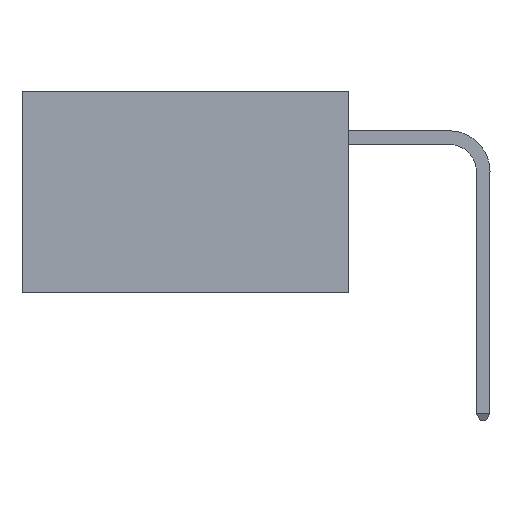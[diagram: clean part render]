
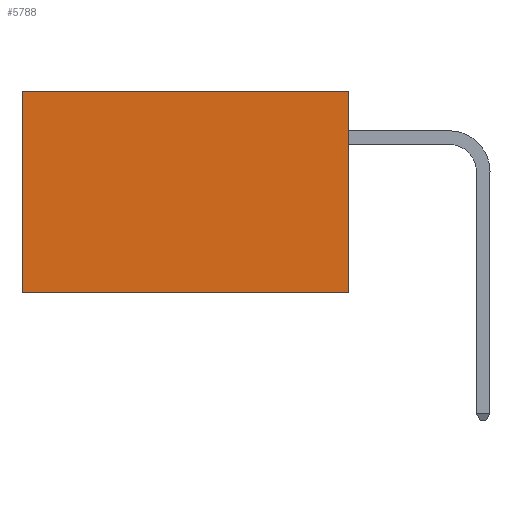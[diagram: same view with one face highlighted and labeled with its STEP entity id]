
A CAD part, left-side view. The second image highlights one B-rep face of the part: STEP entity #5788.
In plain terms, the highlighted planar face has unit normal (-1, 0, 0).
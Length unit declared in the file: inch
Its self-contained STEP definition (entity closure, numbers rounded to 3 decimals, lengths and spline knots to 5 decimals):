
#42 = CARTESIAN_POINT ( 'NONE',  ( 0.2875, 0., 0. ) ) ;
#279 = VERTEX_POINT ( 'NONE', #8494 ) ;
#359 = EDGE_CURVE ( 'NONE', #1684, #279, #5317, .T. ) ;
#578 = VERTEX_POINT ( 'NONE', #4209 ) ;
#621 = CARTESIAN_POINT ( 'NONE',  ( 0.2875, 0., 0. ) ) ;
#719 = DIRECTION ( 'NONE',  ( 0., 1., 0. ) ) ;
#857 = VERTEX_POINT ( 'NONE', #935 ) ;
#935 = CARTESIAN_POINT ( 'NONE',  ( 0.2875, 0.6, -0.37 ) ) ;
#992 = DIRECTION ( 'NONE',  ( 0., 0., -1. ) ) ;
#1509 = VECTOR ( 'NONE', #719, 39.37008 ) ;
#1549 = VECTOR ( 'NONE', #4311, 39.37008 ) ;
#1573 = LINE ( 'NONE', #8195, #1549 ) ;
#1684 = VERTEX_POINT ( 'NONE', #9996 ) ;
#1846 = LINE ( 'NONE', #9400, #1509 ) ;
#1963 = PLANE ( 'NONE',  #2991 ) ;
#2649 = EDGE_CURVE ( 'NONE', #279, #857, #1573, .T. ) ;
#2658 = EDGE_CURVE ( 'NONE', #578, #857, #1846, .T. ) ;
#2991 = AXIS2_PLACEMENT_3D ( 'NONE', #10996, #6759, #992 ) ;
#4039 = EDGE_CURVE ( 'NONE', #1684, #578, #6364, .T. ) ;
#4209 = CARTESIAN_POINT ( 'NONE',  ( 0.2875, 0., -0.37 ) ) ;
#4267 = ORIENTED_EDGE ( 'NONE', *, *, #359, .T. ) ;
#4311 = DIRECTION ( 'NONE',  ( 0., 0., -1. ) ) ;
#4889 = ORIENTED_EDGE ( 'NONE', *, *, #4039, .F. ) ;
#4931 = ORIENTED_EDGE ( 'NONE', *, *, #2658, .F. ) ;
#5108 = VECTOR ( 'NONE', #6990, 39.37008 ) ;
#5241 = ORIENTED_EDGE ( 'NONE', *, *, #2649, .T. ) ;
#5317 = LINE ( 'NONE', #42, #5108 ) ;
#5788 = ADVANCED_FACE ( 'NONE', ( #9772 ), #1963, .F. ) ;
#6364 = LINE ( 'NONE', #621, #8157 ) ;
#6759 = DIRECTION ( 'NONE',  ( 1., 0., 0. ) ) ;
#6990 = DIRECTION ( 'NONE',  ( 0., 1., 0. ) ) ;
#8045 = DIRECTION ( 'NONE',  ( 0., 0., -1. ) ) ;
#8157 = VECTOR ( 'NONE', #8045, 39.37008 ) ;
#8195 = CARTESIAN_POINT ( 'NONE',  ( 0.2875, 0.6, 0. ) ) ;
#8494 = CARTESIAN_POINT ( 'NONE',  ( 0.2875, 0.6, 0. ) ) ;
#8698 = EDGE_LOOP ( 'NONE', ( #5241, #4931, #4889, #4267 ) ) ;
#9400 = CARTESIAN_POINT ( 'NONE',  ( 0.2875, 0., -0.37 ) ) ;
#9772 = FACE_OUTER_BOUND ( 'NONE', #8698, .T. ) ;
#9996 = CARTESIAN_POINT ( 'NONE',  ( 0.2875, 0., 0. ) ) ;
#10996 = CARTESIAN_POINT ( 'NONE',  ( 0.2875, 0., 0. ) ) ;
